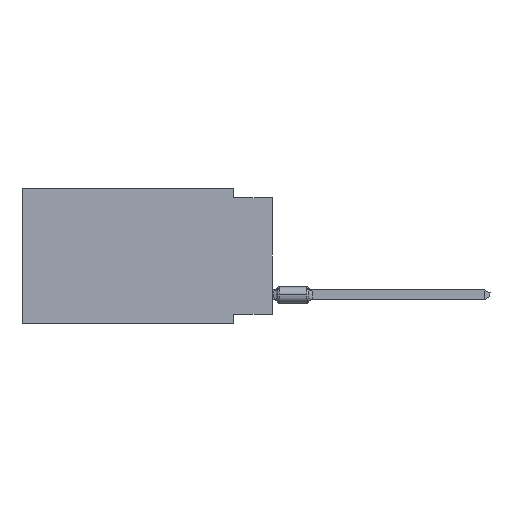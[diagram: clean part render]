
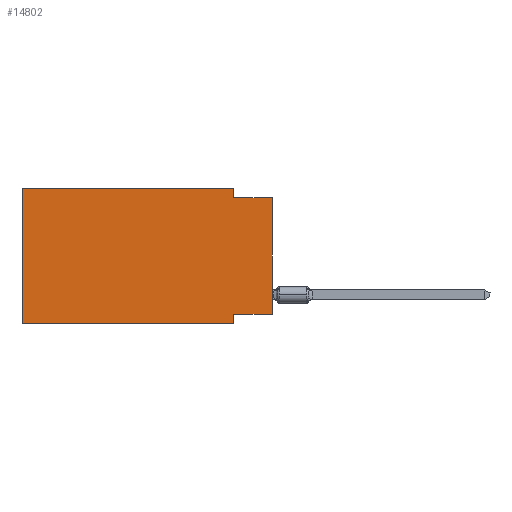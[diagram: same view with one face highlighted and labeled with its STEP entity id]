
A CAD part, left-side view. The second image highlights one B-rep face of the part: STEP entity #14802.
In plain terms, the highlighted planar face has unit normal (-1, 0, 0).
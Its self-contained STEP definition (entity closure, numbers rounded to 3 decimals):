
#396 = VECTOR ( 'NONE', #49346, 1000. ) ;
#1078 = ORIENTED_EDGE ( 'NONE', *, *, #32812, .T. ) ;
#4690 = ORIENTED_EDGE ( 'NONE', *, *, #70033, .F. ) ;
#8539 = LINE ( 'NONE', #68754, #63689 ) ;
#8895 = DIRECTION ( 'NONE',  ( 0., 0., -1. ) ) ;
#10684 = DIRECTION ( 'NONE',  ( 0., 1., 0. ) ) ;
#11989 = VERTEX_POINT ( 'NONE', #52943 ) ;
#12192 = CARTESIAN_POINT ( 'NONE',  ( 0., 2.54, -8.89 ) ) ;
#13591 = EDGE_CURVE ( 'NONE', #38754, #49559, #28803, .T. ) ;
#14301 = EDGE_CURVE ( 'NONE', #11989, #41564, #65251, .T. ) ;
#14600 = ORIENTED_EDGE ( 'NONE', *, *, #30536, .F. ) ;
#14802 = ADVANCED_FACE ( 'NONE', ( #28861 ), #46749, .F. ) ;
#15362 = DIRECTION ( 'NONE',  ( 0., -1., 0. ) ) ;
#15375 = CARTESIAN_POINT ( 'NONE',  ( 0., 0., 0. ) ) ;
#15964 = ORIENTED_EDGE ( 'NONE', *, *, #33573, .F. ) ;
#17079 = EDGE_CURVE ( 'NONE', #49523, #54920, #48004, .T. ) ;
#17927 = DIRECTION ( 'NONE',  ( 0., 0., -1. ) ) ;
#19581 = CARTESIAN_POINT ( 'NONE',  ( 0., 2.54, 0. ) ) ;
#20118 = CARTESIAN_POINT ( 'NONE',  ( 0., 0., -0.635 ) ) ;
#22549 = VECTOR ( 'NONE', #10684, 1000. ) ;
#25282 = EDGE_LOOP ( 'NONE', ( #52162, #14600, #4690, #15964, #27515, #1078, #48892, #52248 ) ) ;
#27168 = LINE ( 'NONE', #54061, #22549 ) ;
#27515 = ORIENTED_EDGE ( 'NONE', *, *, #13591, .F. ) ;
#27814 = VECTOR ( 'NONE', #15362, 1000. ) ;
#28089 = DIRECTION ( 'NONE',  ( 0., 0., 1. ) ) ;
#28530 = LINE ( 'NONE', #45026, #396 ) ;
#28803 = LINE ( 'NONE', #60359, #42511 ) ;
#28861 = FACE_OUTER_BOUND ( 'NONE', #25282, .T. ) ;
#29192 = LINE ( 'NONE', #40303, #67592 ) ;
#30536 = EDGE_CURVE ( 'NONE', #39385, #54920, #29192, .T. ) ;
#32812 = EDGE_CURVE ( 'NONE', #38754, #41564, #42950, .T. ) ;
#33573 = EDGE_CURVE ( 'NONE', #49559, #57556, #28530, .T. ) ;
#34301 = CARTESIAN_POINT ( 'NONE',  ( 0., 16.383, -8.89 ) ) ;
#34574 = CARTESIAN_POINT ( 'NONE',  ( 0., 2.54, -0.635 ) ) ;
#37246 = DIRECTION ( 'NONE',  ( 0., 0., 1. ) ) ;
#38754 = VERTEX_POINT ( 'NONE', #34301 ) ;
#39385 = VERTEX_POINT ( 'NONE', #34574 ) ;
#40303 = CARTESIAN_POINT ( 'NONE',  ( 0., 0., -0.635 ) ) ;
#40316 = DIRECTION ( 'NONE',  ( 0., 0., -1. ) ) ;
#41564 = VERTEX_POINT ( 'NONE', #52360 ) ;
#42511 = VECTOR ( 'NONE', #28089, 1000. ) ;
#42950 = LINE ( 'NONE', #64472, #27814 ) ;
#43733 = VECTOR ( 'NONE', #17927, 1000. ) ;
#45026 = CARTESIAN_POINT ( 'NONE',  ( 0., 16.383, 0. ) ) ;
#46749 = PLANE ( 'NONE',  #50662 ) ;
#48004 = LINE ( 'NONE', #15375, #48542 ) ;
#48542 = VECTOR ( 'NONE', #37246, 1000. ) ;
#48892 = ORIENTED_EDGE ( 'NONE', *, *, #14301, .F. ) ;
#49266 = CARTESIAN_POINT ( 'NONE',  ( 0., 0., -8.255 ) ) ;
#49346 = DIRECTION ( 'NONE',  ( 0., -1., 0. ) ) ;
#49523 = VERTEX_POINT ( 'NONE', #49266 ) ;
#49559 = VERTEX_POINT ( 'NONE', #66103 ) ;
#50662 = AXIS2_PLACEMENT_3D ( 'NONE', #67914, #56810, #40316 ) ;
#52162 = ORIENTED_EDGE ( 'NONE', *, *, #17079, .T. ) ;
#52248 = ORIENTED_EDGE ( 'NONE', *, *, #58577, .F. ) ;
#52360 = CARTESIAN_POINT ( 'NONE',  ( 0., 2.54, -8.89 ) ) ;
#52943 = CARTESIAN_POINT ( 'NONE',  ( 0., 2.54, -8.255 ) ) ;
#54061 = CARTESIAN_POINT ( 'NONE',  ( 0., 0., -8.255 ) ) ;
#54920 = VERTEX_POINT ( 'NONE', #20118 ) ;
#55388 = DIRECTION ( 'NONE',  ( 0., -1., 0. ) ) ;
#56810 = DIRECTION ( 'NONE',  ( 1., 0., 0. ) ) ;
#57556 = VERTEX_POINT ( 'NONE', #19581 ) ;
#58577 = EDGE_CURVE ( 'NONE', #49523, #11989, #27168, .T. ) ;
#60359 = CARTESIAN_POINT ( 'NONE',  ( 0., 16.383, 0. ) ) ;
#63689 = VECTOR ( 'NONE', #8895, 1000. ) ;
#64472 = CARTESIAN_POINT ( 'NONE',  ( 0., 16.383, -8.89 ) ) ;
#65251 = LINE ( 'NONE', #12192, #43733 ) ;
#66103 = CARTESIAN_POINT ( 'NONE',  ( 0., 16.383, 0. ) ) ;
#67592 = VECTOR ( 'NONE', #55388, 1000. ) ;
#67914 = CARTESIAN_POINT ( 'NONE',  ( 0., 16.383, 0. ) ) ;
#68754 = CARTESIAN_POINT ( 'NONE',  ( 0., 2.54, 0. ) ) ;
#70033 = EDGE_CURVE ( 'NONE', #57556, #39385, #8539, .T. ) ;
